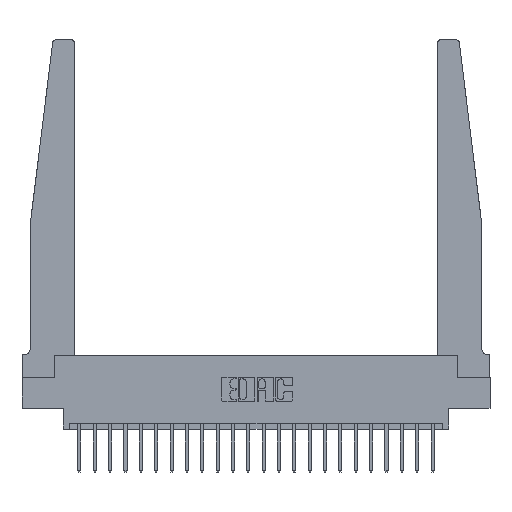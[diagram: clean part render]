
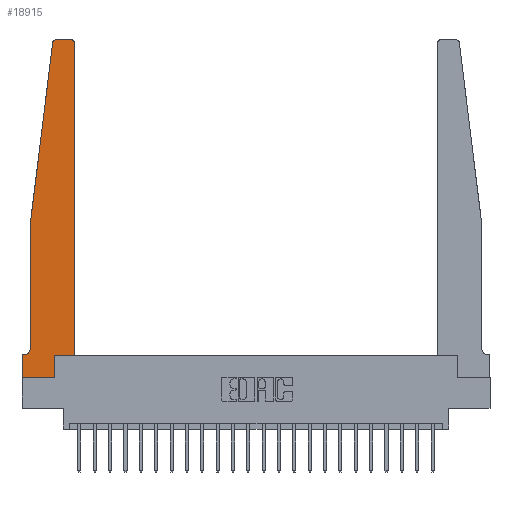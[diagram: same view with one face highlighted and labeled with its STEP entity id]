
A CAD part, top view. The second image highlights one B-rep face of the part: STEP entity #18915.
In plain terms, the highlighted planar face has unit normal (0, 0, 1).
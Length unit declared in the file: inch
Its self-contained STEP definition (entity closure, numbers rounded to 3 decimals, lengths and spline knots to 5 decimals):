
#27 = EDGE_CURVE ( 'NONE', #9375, #21922, #17574, .T. ) ;
#363 = CARTESIAN_POINT ( 'NONE',  ( 0., 0., 0.37 ) ) ;
#1351 = EDGE_CURVE ( 'NONE', #20956, #2124, #7212, .T. ) ;
#1527 = VECTOR ( 'NONE', #6725, 39.37008 ) ;
#1744 = DIRECTION ( 'NONE',  ( 0., 0., 1. ) ) ;
#1894 = VECTOR ( 'NONE', #10746, 39.37008 ) ;
#2124 = VERTEX_POINT ( 'NONE', #12620 ) ;
#2151 = DIRECTION ( 'NONE',  ( 0., -1., 0. ) ) ;
#2194 = ORIENTED_EDGE ( 'NONE', *, *, #11874, .T. ) ;
#2306 = ORIENTED_EDGE ( 'NONE', *, *, #10807, .T. ) ;
#2367 = CARTESIAN_POINT ( 'NONE',  ( 0.425, 0.18, 0.37 ) ) ;
#2854 = CARTESIAN_POINT ( 'NONE',  ( 0.065, 0.2375, 0.37 ) ) ;
#3145 = LINE ( 'NONE', #4041, #12667 ) ;
#3318 = CIRCLE ( 'NONE', #20025, 0.03 ) ;
#4041 = CARTESIAN_POINT ( 'NONE',  ( 0., 0., 0.37 ) ) ;
#5186 = VECTOR ( 'NONE', #20854, 39.37008 ) ;
#5216 = VERTEX_POINT ( 'NONE', #16540 ) ;
#5954 = ORIENTED_EDGE ( 'NONE', *, *, #21295, .T. ) ;
#5985 = DIRECTION ( 'NONE',  ( 0., 0., 1. ) ) ;
#6575 = CIRCLE ( 'NONE', #21473, 0.05 ) ;
#6725 = DIRECTION ( 'NONE',  ( 0., -1., 0. ) ) ;
#6823 = LINE ( 'NONE', #19191, #1527 ) ;
#6824 = CARTESIAN_POINT ( 'NONE',  ( 0.425, 2.72, 0.37 ) ) ;
#6987 = EDGE_CURVE ( 'NONE', #5216, #19059, #3318, .T. ) ;
#7007 = CARTESIAN_POINT ( 'NONE',  ( 0.015, 0.2375, 0.37 ) ) ;
#7077 = VECTOR ( 'NONE', #21358, 39.37008 ) ;
#7174 = CARTESIAN_POINT ( 'NONE',  ( 0.065, 1.25, 0.37 ) ) ;
#7212 = LINE ( 'NONE', #16645, #21430 ) ;
#7266 = CARTESIAN_POINT ( 'NONE',  ( 0.425, 0.18, 0.37 ) ) ;
#7556 = CARTESIAN_POINT ( 'NONE',  ( 0.2605, 0., 0.37 ) ) ;
#7598 = CARTESIAN_POINT ( 'NONE',  ( 0.27653, 2.72, 0.37 ) ) ;
#7614 = ORIENTED_EDGE ( 'NONE', *, *, #14249, .T. ) ;
#7801 = VERTEX_POINT ( 'NONE', #15510 ) ;
#7820 = LINE ( 'NONE', #7174, #20891 ) ;
#8455 = VERTEX_POINT ( 'NONE', #18918 ) ;
#8603 = FACE_OUTER_BOUND ( 'NONE', #21269, .T. ) ;
#8822 = DIRECTION ( 'NONE',  ( -1., 0., 0. ) ) ;
#8992 = VERTEX_POINT ( 'NONE', #2854 ) ;
#9001 = ORIENTED_EDGE ( 'NONE', *, *, #14092, .T. ) ;
#9375 = VERTEX_POINT ( 'NONE', #2367 ) ;
#9424 = DIRECTION ( 'NONE',  ( 1., 0., 0. ) ) ;
#10566 = EDGE_CURVE ( 'NONE', #7801, #8455, #22385, .T. ) ;
#10746 = DIRECTION ( 'NONE',  ( -1., 0., 0. ) ) ;
#10807 = EDGE_CURVE ( 'NONE', #8455, #20956, #3145, .T. ) ;
#10818 = DIRECTION ( 'NONE',  ( -0.122, -0.992, 0. ) ) ;
#10969 = CARTESIAN_POINT ( 'NONE',  ( 0.065, 0.1875, 0.37 ) ) ;
#11288 = CARTESIAN_POINT ( 'NONE',  ( 0.395, 2.75, 0.37 ) ) ;
#11322 = DIRECTION ( 'NONE',  ( 0., 1., 0. ) ) ;
#11874 = EDGE_CURVE ( 'NONE', #14046, #7801, #15568, .T. ) ;
#12446 = CIRCLE ( 'NONE', #13682, 0.03 ) ;
#12462 = CARTESIAN_POINT ( 'NONE',  ( 0., 0.1875, 0.37 ) ) ;
#12620 = CARTESIAN_POINT ( 'NONE',  ( 0.2605, 0.18, 0.37 ) ) ;
#12667 = VECTOR ( 'NONE', #16495, 39.37008 ) ;
#12842 = CARTESIAN_POINT ( 'NONE',  ( 0.24675, 2.72367, 0.37 ) ) ;
#12937 = CARTESIAN_POINT ( 'NONE',  ( 0.065, 1.25, 0.37 ) ) ;
#13010 = AXIS2_PLACEMENT_3D ( 'NONE', #12462, #1744, #14228 ) ;
#13351 = ORIENTED_EDGE ( 'NONE', *, *, #17594, .T. ) ;
#13458 = ORIENTED_EDGE ( 'NONE', *, *, #6987, .T. ) ;
#13682 = AXIS2_PLACEMENT_3D ( 'NONE', #16630, #5985, #18423 ) ;
#13712 = VERTEX_POINT ( 'NONE', #12937 ) ;
#13791 = EDGE_CURVE ( 'NONE', #21922, #20402, #12446, .T. ) ;
#14046 = VERTEX_POINT ( 'NONE', #17242 ) ;
#14092 = EDGE_CURVE ( 'NONE', #13712, #8992, #6823, .T. ) ;
#14228 = DIRECTION ( 'NONE',  ( 1., 0., 0. ) ) ;
#14249 = EDGE_CURVE ( 'NONE', #20402, #5216, #21304, .T. ) ;
#15510 = CARTESIAN_POINT ( 'NONE',  ( 0., 0.1875, 0.37 ) ) ;
#15568 = LINE ( 'NONE', #10969, #1894 ) ;
#16495 = DIRECTION ( 'NONE',  ( 1., 0., 0. ) ) ;
#16540 = CARTESIAN_POINT ( 'NONE',  ( 0.27653, 2.75, 0.37 ) ) ;
#16630 = CARTESIAN_POINT ( 'NONE',  ( 0.395, 2.72, 0.37 ) ) ;
#16645 = CARTESIAN_POINT ( 'NONE',  ( 0.2605, 0.18, 0.37 ) ) ;
#17242 = CARTESIAN_POINT ( 'NONE',  ( 0.015, 0.1875, 0.37 ) ) ;
#17574 = LINE ( 'NONE', #7266, #21759 ) ;
#17594 = EDGE_CURVE ( 'NONE', #19059, #13712, #7820, .T. ) ;
#17622 = ORIENTED_EDGE ( 'NONE', *, *, #1351, .T. ) ;
#18225 = ORIENTED_EDGE ( 'NONE', *, *, #20739, .T. ) ;
#18423 = DIRECTION ( 'NONE',  ( 1., 0., 0. ) ) ;
#18915 = ADVANCED_FACE ( 'NONE', ( #8603 ), #19503, .T. ) ;
#18918 = CARTESIAN_POINT ( 'NONE',  ( 0., 0., 0.37 ) ) ;
#19059 = VERTEX_POINT ( 'NONE', #12842 ) ;
#19191 = CARTESIAN_POINT ( 'NONE',  ( 0.065, 1.25, 0.37 ) ) ;
#19402 = LINE ( 'NONE', #22546, #5186 ) ;
#19476 = DIRECTION ( 'NONE',  ( 0., 0., -1. ) ) ;
#19503 = PLANE ( 'NONE',  #13010 ) ;
#19565 = CARTESIAN_POINT ( 'NONE',  ( 0.25, 2.75, 0.37 ) ) ;
#19654 = DIRECTION ( 'NONE',  ( 0., 1., 0. ) ) ;
#20025 = AXIS2_PLACEMENT_3D ( 'NONE', #7598, #20043, #9424 ) ;
#20043 = DIRECTION ( 'NONE',  ( 0., 0., 1. ) ) ;
#20045 = ORIENTED_EDGE ( 'NONE', *, *, #10566, .T. ) ;
#20402 = VERTEX_POINT ( 'NONE', #11288 ) ;
#20739 = EDGE_CURVE ( 'NONE', #8992, #14046, #6575, .T. ) ;
#20763 = ORIENTED_EDGE ( 'NONE', *, *, #27, .T. ) ;
#20854 = DIRECTION ( 'NONE',  ( 1., 0., 0. ) ) ;
#20891 = VECTOR ( 'NONE', #10818, 39.37008 ) ;
#20956 = VERTEX_POINT ( 'NONE', #7556 ) ;
#21269 = EDGE_LOOP ( 'NONE', ( #7614, #13458, #13351, #9001, #18225, #2194, #20045, #2306, #17622, #5954, #20763, #22956 ) ) ;
#21273 = VECTOR ( 'NONE', #2151, 39.37008 ) ;
#21295 = EDGE_CURVE ( 'NONE', #2124, #9375, #19402, .T. ) ;
#21304 = LINE ( 'NONE', #19565, #7077 ) ;
#21358 = DIRECTION ( 'NONE',  ( -1., 0., 0. ) ) ;
#21430 = VECTOR ( 'NONE', #11322, 39.37008 ) ;
#21473 = AXIS2_PLACEMENT_3D ( 'NONE', #7007, #19476, #8822 ) ;
#21759 = VECTOR ( 'NONE', #19654, 39.37008 ) ;
#21922 = VERTEX_POINT ( 'NONE', #6824 ) ;
#22385 = LINE ( 'NONE', #363, #21273 ) ;
#22546 = CARTESIAN_POINT ( 'NONE',  ( 0.425, 0.18, 0.37 ) ) ;
#22956 = ORIENTED_EDGE ( 'NONE', *, *, #13791, .T. ) ;
